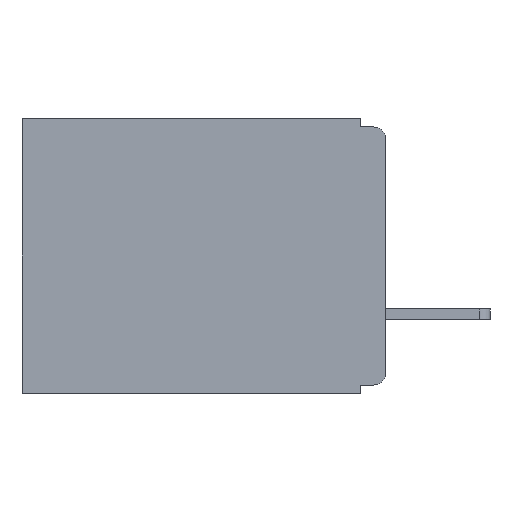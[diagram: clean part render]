
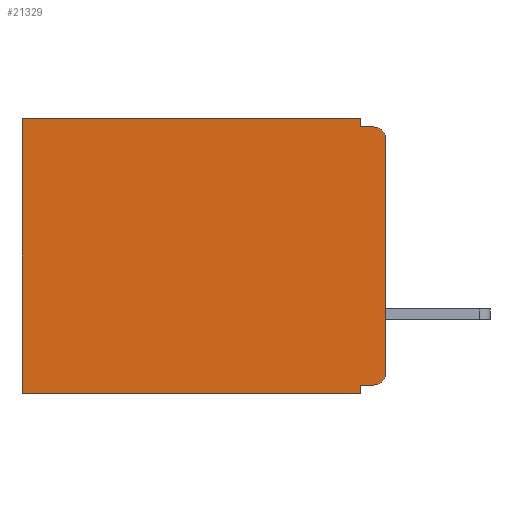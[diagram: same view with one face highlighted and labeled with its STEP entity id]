
A CAD part, left-side view. The second image highlights one B-rep face of the part: STEP entity #21329.
In plain terms, the highlighted planar face has unit normal (-1, 0, 0).
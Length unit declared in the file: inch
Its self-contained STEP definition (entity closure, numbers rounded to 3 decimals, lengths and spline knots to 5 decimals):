
#367 = AXIS2_PLACEMENT_3D ( 'NONE', #843, #13270, #2633 ) ;
#568 = ORIENTED_EDGE ( 'NONE', *, *, #22900, .F. ) ;
#607 = PLANE ( 'NONE',  #15498 ) ;
#843 = CARTESIAN_POINT ( 'NONE',  ( 0.3, 0.015, -0.305 ) ) ;
#1275 = LINE ( 'NONE', #1677, #10179 ) ;
#1562 = CARTESIAN_POINT ( 'NONE',  ( 0.3, 0.437, 0. ) ) ;
#1639 = EDGE_CURVE ( 'NONE', #2461, #18363, #22870, .T. ) ;
#1677 = CARTESIAN_POINT ( 'NONE',  ( 0.3, 0., 0. ) ) ;
#2394 = DIRECTION ( 'NONE',  ( 1., 0., 0. ) ) ;
#2442 = VERTEX_POINT ( 'NONE', #6482 ) ;
#2461 = VERTEX_POINT ( 'NONE', #14375 ) ;
#2521 = VECTOR ( 'NONE', #16203, 39.37008 ) ;
#2530 = CARTESIAN_POINT ( 'NONE',  ( 0.3, 0.031, 0. ) ) ;
#2633 = DIRECTION ( 'NONE',  ( 0., 0., -1. ) ) ;
#3097 = CARTESIAN_POINT ( 'NONE',  ( 0.3, 0.015, -0.01 ) ) ;
#3123 = EDGE_CURVE ( 'NONE', #6907, #21761, #17756, .T. ) ;
#3194 = CARTESIAN_POINT ( 'NONE',  ( 0.3, 0., -0.305 ) ) ;
#3319 = CARTESIAN_POINT ( 'NONE',  ( 0.3, 0.437, -0.33 ) ) ;
#3452 = DIRECTION ( 'NONE',  ( 0., 1., 0. ) ) ;
#3558 = CARTESIAN_POINT ( 'NONE',  ( 0.3, 0., -0.33 ) ) ;
#3575 = VECTOR ( 'NONE', #19683, 39.37008 ) ;
#5129 = DIRECTION ( 'NONE',  ( 0., 0., -1. ) ) ;
#6482 = CARTESIAN_POINT ( 'NONE',  ( 0.3, 0.031, -0.01 ) ) ;
#6619 = CARTESIAN_POINT ( 'NONE',  ( 0.3, 0.437, -0.33 ) ) ;
#6806 = ORIENTED_EDGE ( 'NONE', *, *, #17357, .F. ) ;
#6860 = ORIENTED_EDGE ( 'NONE', *, *, #16060, .F. ) ;
#6907 = VERTEX_POINT ( 'NONE', #22504 ) ;
#7283 = VERTEX_POINT ( 'NONE', #6619 ) ;
#7409 = CARTESIAN_POINT ( 'NONE',  ( 0.3, 0., -0.01 ) ) ;
#7414 = VECTOR ( 'NONE', #17491, 39.37008 ) ;
#7745 = ORIENTED_EDGE ( 'NONE', *, *, #21939, .T. ) ;
#7897 = FACE_OUTER_BOUND ( 'NONE', #14948, .T. ) ;
#8199 = CARTESIAN_POINT ( 'NONE',  ( 0.3, 0.031, -0.33 ) ) ;
#8723 = ORIENTED_EDGE ( 'NONE', *, *, #19848, .T. ) ;
#8799 = DIRECTION ( 'NONE',  ( -1., 0., 0. ) ) ;
#9240 = LINE ( 'NONE', #3319, #18154 ) ;
#9517 = DIRECTION ( 'NONE',  ( 0., 0., -1. ) ) ;
#9829 = ORIENTED_EDGE ( 'NONE', *, *, #22542, .T. ) ;
#10179 = VECTOR ( 'NONE', #3452, 39.37008 ) ;
#11502 = DIRECTION ( 'NONE',  ( 0., 1., 0. ) ) ;
#11589 = CARTESIAN_POINT ( 'NONE',  ( 0.3, 0.031, -0.33 ) ) ;
#11978 = LINE ( 'NONE', #14414, #2521 ) ;
#12246 = ORIENTED_EDGE ( 'NONE', *, *, #3123, .F. ) ;
#12350 = CIRCLE ( 'NONE', #367, 0.015 ) ;
#12361 = VERTEX_POINT ( 'NONE', #3097 ) ;
#12405 = EDGE_CURVE ( 'NONE', #14727, #6907, #13227, .T. ) ;
#12410 = VERTEX_POINT ( 'NONE', #1562 ) ;
#13017 = CARTESIAN_POINT ( 'NONE',  ( 0.3, 0., -0.33 ) ) ;
#13227 = LINE ( 'NONE', #21075, #7414 ) ;
#13270 = DIRECTION ( 'NONE',  ( -1., 0., 0. ) ) ;
#13350 = VECTOR ( 'NONE', #21633, 39.37008 ) ;
#14141 = EDGE_CURVE ( 'NONE', #14727, #18363, #12350, .T. ) ;
#14185 = ORIENTED_EDGE ( 'NONE', *, *, #14141, .T. ) ;
#14375 = CARTESIAN_POINT ( 'NONE',  ( 0.3, 0., -0.025 ) ) ;
#14414 = CARTESIAN_POINT ( 'NONE',  ( 0.3, 0.031, 0. ) ) ;
#14727 = VERTEX_POINT ( 'NONE', #14946 ) ;
#14804 = DIRECTION ( 'NONE',  ( 0., 0., -1. ) ) ;
#14946 = CARTESIAN_POINT ( 'NONE',  ( 0.3, 0.015, -0.32 ) ) ;
#14948 = EDGE_LOOP ( 'NONE', ( #16264, #7745, #6806, #6860, #8723, #9829, #568, #12246, #19197, #14185 ) ) ;
#15051 = LINE ( 'NONE', #16771, #15596 ) ;
#15498 = AXIS2_PLACEMENT_3D ( 'NONE', #13017, #2394, #14804 ) ;
#15596 = VECTOR ( 'NONE', #11502, 39.37008 ) ;
#15880 = CIRCLE ( 'NONE', #17319, 0.015 ) ;
#16060 = EDGE_CURVE ( 'NONE', #21655, #2442, #11978, .T. ) ;
#16203 = DIRECTION ( 'NONE',  ( 0., 0., -1. ) ) ;
#16264 = ORIENTED_EDGE ( 'NONE', *, *, #1639, .F. ) ;
#16771 = CARTESIAN_POINT ( 'NONE',  ( 0.3, 0., -0.33 ) ) ;
#17319 = AXIS2_PLACEMENT_3D ( 'NONE', #19460, #8799, #21252 ) ;
#17357 = EDGE_CURVE ( 'NONE', #2442, #12361, #22830, .T. ) ;
#17491 = DIRECTION ( 'NONE',  ( 0., 1., 0. ) ) ;
#17756 = LINE ( 'NONE', #11589, #3575 ) ;
#18154 = VECTOR ( 'NONE', #5129, 39.37008 ) ;
#18363 = VERTEX_POINT ( 'NONE', #3194 ) ;
#19197 = ORIENTED_EDGE ( 'NONE', *, *, #12405, .F. ) ;
#19460 = CARTESIAN_POINT ( 'NONE',  ( 0.3, 0.015, -0.025 ) ) ;
#19683 = DIRECTION ( 'NONE',  ( 0., 0., -1. ) ) ;
#19848 = EDGE_CURVE ( 'NONE', #21655, #12410, #1275, .T. ) ;
#21075 = CARTESIAN_POINT ( 'NONE',  ( 0.3, 0., -0.32 ) ) ;
#21252 = DIRECTION ( 'NONE',  ( 0., 0., -1. ) ) ;
#21329 = ADVANCED_FACE ( 'NONE', ( #7897 ), #607, .F. ) ;
#21633 = DIRECTION ( 'NONE',  ( 0., -1., 0. ) ) ;
#21655 = VERTEX_POINT ( 'NONE', #2530 ) ;
#21761 = VERTEX_POINT ( 'NONE', #8199 ) ;
#21939 = EDGE_CURVE ( 'NONE', #2461, #12361, #15880, .T. ) ;
#22312 = VECTOR ( 'NONE', #9517, 39.37008 ) ;
#22504 = CARTESIAN_POINT ( 'NONE',  ( 0.3, 0.031, -0.32 ) ) ;
#22542 = EDGE_CURVE ( 'NONE', #12410, #7283, #9240, .T. ) ;
#22830 = LINE ( 'NONE', #7409, #13350 ) ;
#22870 = LINE ( 'NONE', #3558, #22312 ) ;
#22900 = EDGE_CURVE ( 'NONE', #21761, #7283, #15051, .T. ) ;
